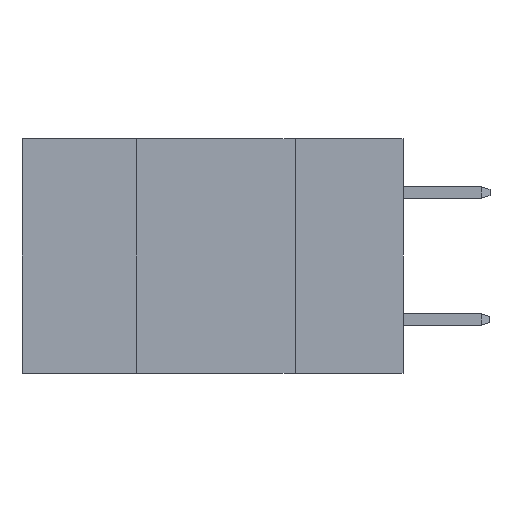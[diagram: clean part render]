
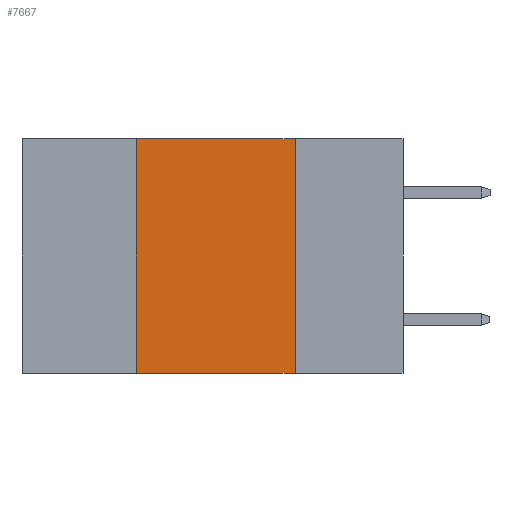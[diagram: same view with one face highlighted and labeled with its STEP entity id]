
A CAD part, left-side view. The second image highlights one B-rep face of the part: STEP entity #7667.
In plain terms, the highlighted planar face has unit normal (-1, 0, 0).
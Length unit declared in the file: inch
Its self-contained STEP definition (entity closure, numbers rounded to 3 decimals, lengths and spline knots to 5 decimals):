
#740 = PLANE ( 'NONE',  #6802 ) ;
#744 = VERTEX_POINT ( 'NONE', #5749 ) ;
#1080 = VERTEX_POINT ( 'NONE', #7618 ) ;
#1371 = LINE ( 'NONE', #3511, #2183 ) ;
#2121 = VERTEX_POINT ( 'NONE', #8458 ) ;
#2128 = EDGE_CURVE ( 'NONE', #2121, #1080, #1371, .T. ) ;
#2175 = EDGE_CURVE ( 'NONE', #2121, #744, #12554, .T. ) ;
#2177 = EDGE_CURVE ( 'NONE', #744, #2590, #9756, .T. ) ;
#2183 = VECTOR ( 'NONE', #9327, 39.37008 ) ;
#2395 = VECTOR ( 'NONE', #10747, 39.37008 ) ;
#2458 = LINE ( 'NONE', #10415, #4267 ) ;
#2512 = EDGE_CURVE ( 'NONE', #2590, #1080, #2458, .T. ) ;
#2590 = VERTEX_POINT ( 'NONE', #9936 ) ;
#2691 = DIRECTION ( 'NONE',  ( 1., 0., 0. ) ) ;
#3511 = CARTESIAN_POINT ( 'NONE',  ( 0., 0.6, -0.37 ) ) ;
#3761 = DIRECTION ( 'NONE',  ( 0., -1., 0. ) ) ;
#4267 = VECTOR ( 'NONE', #11688, 39.37008 ) ;
#4673 = DIRECTION ( 'NONE',  ( 0., 0., -1. ) ) ;
#5275 = VECTOR ( 'NONE', #3761, 39.37008 ) ;
#5700 = ORIENTED_EDGE ( 'NONE', *, *, #2128, .T. ) ;
#5749 = CARTESIAN_POINT ( 'NONE',  ( 0., 0.42, 0. ) ) ;
#6769 = CARTESIAN_POINT ( 'NONE',  ( 0., 0.6, 0. ) ) ;
#6802 = AXIS2_PLACEMENT_3D ( 'NONE', #11512, #2691, #4673 ) ;
#7618 = CARTESIAN_POINT ( 'NONE',  ( 0., 0.17, -0.37 ) ) ;
#7635 = ORIENTED_EDGE ( 'NONE', *, *, #2177, .F. ) ;
#7667 = ADVANCED_FACE ( 'NONE', ( #11648 ), #740, .F. ) ;
#7777 = CARTESIAN_POINT ( 'NONE',  ( 0., 0.42, 0. ) ) ;
#8458 = CARTESIAN_POINT ( 'NONE',  ( 0., 0.42, -0.37 ) ) ;
#9327 = DIRECTION ( 'NONE',  ( 0., -1., 0. ) ) ;
#9756 = LINE ( 'NONE', #6769, #5275 ) ;
#9936 = CARTESIAN_POINT ( 'NONE',  ( 0., 0.17, 0. ) ) ;
#10415 = CARTESIAN_POINT ( 'NONE',  ( 0., 0.17, 0. ) ) ;
#10747 = DIRECTION ( 'NONE',  ( 0., 0., 1. ) ) ;
#11181 = ORIENTED_EDGE ( 'NONE', *, *, #2175, .F. ) ;
#11438 = ORIENTED_EDGE ( 'NONE', *, *, #2512, .F. ) ;
#11512 = CARTESIAN_POINT ( 'NONE',  ( 0., 0.6, 0. ) ) ;
#11648 = FACE_OUTER_BOUND ( 'NONE', #12685, .T. ) ;
#11688 = DIRECTION ( 'NONE',  ( 0., 0., -1. ) ) ;
#12554 = LINE ( 'NONE', #7777, #2395 ) ;
#12685 = EDGE_LOOP ( 'NONE', ( #11438, #7635, #11181, #5700 ) ) ;
